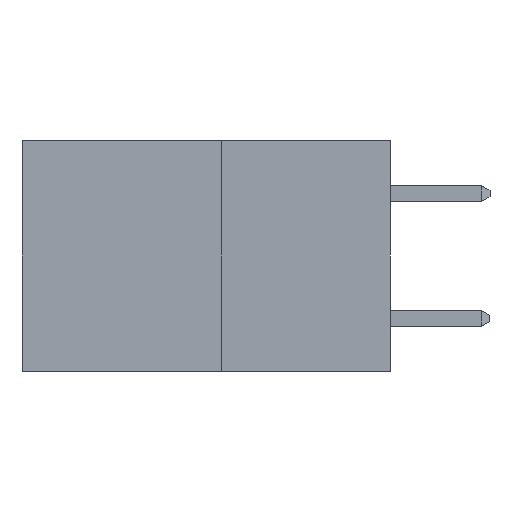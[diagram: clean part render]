
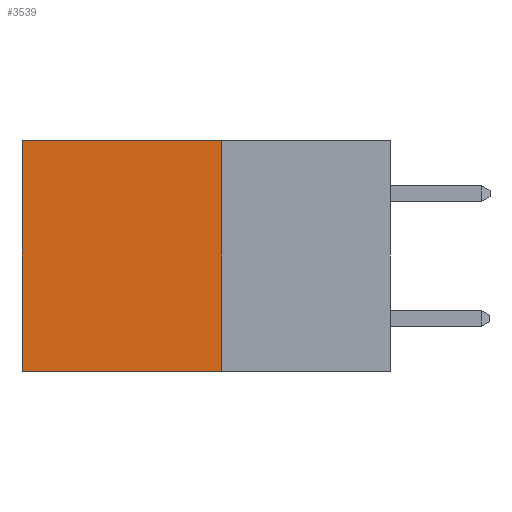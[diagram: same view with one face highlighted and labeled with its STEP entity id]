
A CAD part, left-side view. The second image highlights one B-rep face of the part: STEP entity #3539.
In plain terms, the highlighted planar face has unit normal (-1, 0, 0).
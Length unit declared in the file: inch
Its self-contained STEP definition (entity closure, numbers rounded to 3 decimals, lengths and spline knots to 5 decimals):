
#372 = DIRECTION ( 'NONE',  ( 0., 0., -1. ) ) ;
#892 = EDGE_CURVE ( 'NONE', #4149, #3348, #4736, .T. ) ;
#1131 = ORIENTED_EDGE ( 'NONE', *, *, #5662, .T. ) ;
#1831 = LINE ( 'NONE', #6165, #4813 ) ;
#1986 = CARTESIAN_POINT ( 'NONE',  ( 0.277, 0.27, 0. ) ) ;
#2308 = LINE ( 'NONE', #6663, #6416 ) ;
#2478 = CARTESIAN_POINT ( 'NONE',  ( 0.277, 0.59, -0.37 ) ) ;
#2633 = EDGE_LOOP ( 'NONE', ( #1131, #4279, #3273, #3112 ) ) ;
#3080 = CARTESIAN_POINT ( 'NONE',  ( 0.277, 0.27, 0. ) ) ;
#3112 = ORIENTED_EDGE ( 'NONE', *, *, #892, .T. ) ;
#3168 = PLANE ( 'NONE',  #3336 ) ;
#3199 = VECTOR ( 'NONE', #372, 39.37008 ) ;
#3273 = ORIENTED_EDGE ( 'NONE', *, *, #4400, .F. ) ;
#3336 = AXIS2_PLACEMENT_3D ( 'NONE', #4694, #4381, #4603 ) ;
#3348 = VERTEX_POINT ( 'NONE', #6672 ) ;
#3539 = ADVANCED_FACE ( 'NONE', ( #3847 ), #3168, .F. ) ;
#3733 = EDGE_CURVE ( 'NONE', #5515, #6702, #2308, .T. ) ;
#3808 = DIRECTION ( 'NONE',  ( 0., 1., 0. ) ) ;
#3847 = FACE_OUTER_BOUND ( 'NONE', #2633, .T. ) ;
#4149 = VERTEX_POINT ( 'NONE', #1986 ) ;
#4279 = ORIENTED_EDGE ( 'NONE', *, *, #3733, .F. ) ;
#4381 = DIRECTION ( 'NONE',  ( 1., 0., 0. ) ) ;
#4400 = EDGE_CURVE ( 'NONE', #4149, #5515, #1831, .T. ) ;
#4603 = DIRECTION ( 'NONE',  ( 0., 0., -1. ) ) ;
#4691 = LINE ( 'NONE', #2478, #3199 ) ;
#4694 = CARTESIAN_POINT ( 'NONE',  ( 0.277, 0.27, -0.37 ) ) ;
#4736 = LINE ( 'NONE', #3080, #6612 ) ;
#4813 = VECTOR ( 'NONE', #6133, 39.37008 ) ;
#5217 = DIRECTION ( 'NONE',  ( 0., 1., 0. ) ) ;
#5236 = CARTESIAN_POINT ( 'NONE',  ( 0.277, 0.59, -0.37 ) ) ;
#5310 = CARTESIAN_POINT ( 'NONE',  ( 0.277, 0.27, -0.37 ) ) ;
#5515 = VERTEX_POINT ( 'NONE', #5310 ) ;
#5662 = EDGE_CURVE ( 'NONE', #3348, #6702, #4691, .T. ) ;
#6133 = DIRECTION ( 'NONE',  ( 0., 0., -1. ) ) ;
#6165 = CARTESIAN_POINT ( 'NONE',  ( 0.277, 0.27, -0.37 ) ) ;
#6416 = VECTOR ( 'NONE', #5217, 39.37008 ) ;
#6612 = VECTOR ( 'NONE', #3808, 39.37008 ) ;
#6663 = CARTESIAN_POINT ( 'NONE',  ( 0.277, 0.27, -0.37 ) ) ;
#6672 = CARTESIAN_POINT ( 'NONE',  ( 0.277, 0.59, 0. ) ) ;
#6702 = VERTEX_POINT ( 'NONE', #5236 ) ;
